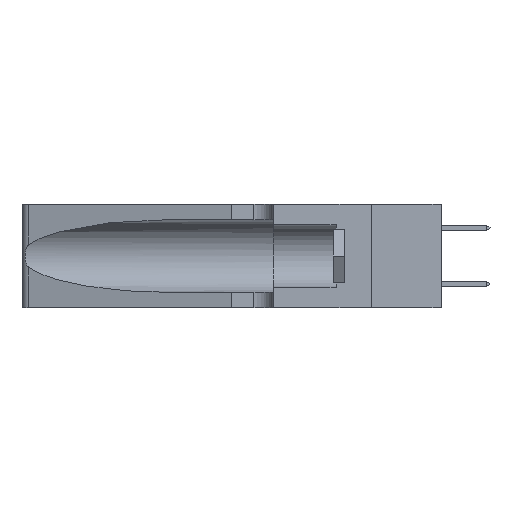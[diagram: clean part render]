
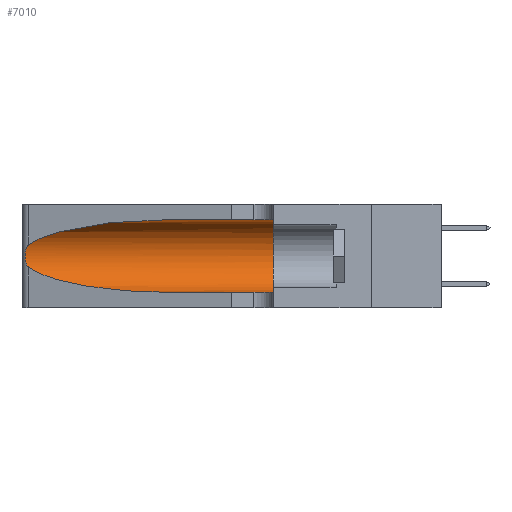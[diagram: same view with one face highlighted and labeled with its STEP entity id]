
A CAD part, left-side view. The second image highlights one B-rep face of the part: STEP entity #7010.
In plain terms, the highlighted cylindrical face has radius 3.308 mm (diameter 6.617 mm), a partial arc.
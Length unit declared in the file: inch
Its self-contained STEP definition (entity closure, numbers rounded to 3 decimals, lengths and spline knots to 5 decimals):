
#22 = CARTESIAN_POINT ( 'NONE',  ( 0.26017, 1.23833, 0.17102 ) ) ;
#208 = ORIENTED_EDGE ( 'NONE', *, *, #18053, .T. ) ;
#286 = VERTEX_POINT ( 'NONE', #5346 ) ;
#726 = EDGE_CURVE ( 'NONE', #14217, #21030, #21893, .T. ) ;
#1141 =( BOUNDED_CURVE ( )  B_SPLINE_CURVE ( 3, ( #11148, #11745, #5069, #12474 ),
 .UNSPECIFIED., .F., .F. ) 
 B_SPLINE_CURVE_WITH_KNOTS ( ( 4, 4 ),
 ( 3.44316, 4.71239 ),
 .UNSPECIFIED. ) 
 CURVE ( )  GEOMETRIC_REPRESENTATION_ITEM ( )  RATIONAL_B_SPLINE_CURVE ( ( 1., 0.87, 0.87, 1. ) ) 
 REPRESENTATION_ITEM ( '' )  );
#1900 = CARTESIAN_POINT ( 'NONE',  ( 0.25787, 1.23484, 0.2124 ) ) ;
#2143 = CARTESIAN_POINT ( 'NONE',  ( 0.26075, 1.23896, 0.19203 ) ) ;
#2318 = VERTEX_POINT ( 'NONE', #16138 ) ;
#2430 = EDGE_CURVE ( 'NONE', #21030, #9475, #13844, .T. ) ;
#3172 = CARTESIAN_POINT ( 'NONE',  ( 0.25487, 1.22718, 0.22369 ) ) ;
#3685 = CARTESIAN_POINT ( 'NONE',  ( 0.25856, 1.23593, 0.16098 ) ) ;
#3752 = CARTESIAN_POINT ( 'NONE',  ( 0.25854, 1.2359, 0.20912 ) ) ;
#3926 = CARTESIAN_POINT ( 'NONE',  ( 0.1305, 0.72297, 0.31525 ) ) ;
#4251 = CARTESIAN_POINT ( 'NONE',  ( 0.25555, 1.22993, 0.14849 ) ) ;
#4576 = CARTESIAN_POINT ( 'NONE',  ( 0.1305, 1.61858, 0.185 ) ) ;
#4674 = ORIENTED_EDGE ( 'NONE', *, *, #5814, .T. ) ;
#4937 = CARTESIAN_POINT ( 'NONE',  ( 0.1305, 1.61858, 0.05475 ) ) ;
#5069 = CARTESIAN_POINT ( 'NONE',  ( 0.18966, 0.96281, 0.05475 ) ) ;
#5147 = EDGE_CURVE ( 'NONE', #286, #2318, #13056, .T. ) ;
#5334 = ORIENTED_EDGE ( 'NONE', *, *, #726, .T. ) ;
#5346 = CARTESIAN_POINT ( 'NONE',  ( 0.1305, 0.35, 0.31525 ) ) ;
#5475 = CARTESIAN_POINT ( 'NONE',  ( 0.2373, 1.15595, 0.28018 ) ) ;
#5515 = CARTESIAN_POINT ( 'NONE',  ( 0.25639, 1.23186, 0.15144 ) ) ;
#5814 = EDGE_CURVE ( 'NONE', #9475, #20450, #1141, .T. ) ;
#7010 = ADVANCED_FACE ( 'NONE', ( #17725 ), #16024, .F. ) ;
#7580 = CARTESIAN_POINT ( 'NONE',  ( 0.25487, 1.22718, 0.22369 ) ) ;
#7705 = CARTESIAN_POINT ( 'NONE',  ( 0.25487, 1.22718, 0.14631 ) ) ;
#8514 = DIRECTION ( 'NONE',  ( 0., -1., 0. ) ) ;
#8834 = LINE ( 'NONE', #20556, #15695 ) ;
#8961 = CARTESIAN_POINT ( 'NONE',  ( 0.1305, 0.72297, 0.31525 ) ) ;
#9475 = VERTEX_POINT ( 'NONE', #7705 ) ;
#10268 = DIRECTION ( 'NONE',  ( 0., 0., 1. ) ) ;
#10344 = DIRECTION ( 'NONE',  ( 0., 1., 0. ) ) ;
#10868 = CARTESIAN_POINT ( 'NONE',  ( 0.25555, 1.22994, 0.2215 ) ) ;
#11148 = CARTESIAN_POINT ( 'NONE',  ( 0.25487, 1.22718, 0.14631 ) ) ;
#11170 = CARTESIAN_POINT ( 'NONE',  ( 0.26018, 1.23835, 0.19895 ) ) ;
#11745 = CARTESIAN_POINT ( 'NONE',  ( 0.2373, 1.15595, 0.08982 ) ) ;
#11842 = CARTESIAN_POINT ( 'NONE',  ( 0.25487, 1.22718, 0.14631 ) ) ;
#12474 = CARTESIAN_POINT ( 'NONE',  ( 0.1305, 0.72297, 0.05475 ) ) ;
#13056 = CIRCLE ( 'NONE', #15812, 0.13025 ) ;
#13256 = CARTESIAN_POINT ( 'NONE',  ( 0.1305, 0.72297, 0.05475 ) ) ;
#13257 = DIRECTION ( 'NONE',  ( 0., -1., 0. ) ) ;
#13844 = B_SPLINE_CURVE_WITH_KNOTS ( 'NONE', 3,
 ( #7580, #10868, #22161, #1900, #3752, #11170, #2143, #21847, #22, #3685, #16455, #5515, #4251, #11842 ),
 .UNSPECIFIED., .F., .F.,
 ( 4, 2, 2, 2, 2, 2, 4 ),
 ( 0., 0.00027, 0.00053, 0.00107, 0.0016, 0.00187, 0.00214 ),
 .UNSPECIFIED. ) ;
#14217 = VERTEX_POINT ( 'NONE', #3926 ) ;
#15176 = ORIENTED_EDGE ( 'NONE', *, *, #2430, .T. ) ;
#15252 = EDGE_LOOP ( 'NONE', ( #5334, #15176, #4674, #208, #22486, #15379 ) ) ;
#15379 = ORIENTED_EDGE ( 'NONE', *, *, #17724, .F. ) ;
#15695 = VECTOR ( 'NONE', #13257, 39.37008 ) ;
#15812 = AXIS2_PLACEMENT_3D ( 'NONE', #19545, #10344, #10268 ) ;
#16024 = CYLINDRICAL_SURFACE ( 'NONE', #16303, 0.13025 ) ;
#16138 = CARTESIAN_POINT ( 'NONE',  ( 0.1305, 0.35, 0.05475 ) ) ;
#16303 = AXIS2_PLACEMENT_3D ( 'NONE', #4576, #20918, #22941 ) ;
#16455 = CARTESIAN_POINT ( 'NONE',  ( 0.25789, 1.23486, 0.15765 ) ) ;
#16554 = CARTESIAN_POINT ( 'NONE',  ( 0.25487, 1.22718, 0.22369 ) ) ;
#17724 = EDGE_CURVE ( 'NONE', #14217, #286, #8834, .T. ) ;
#17725 = FACE_OUTER_BOUND ( 'NONE', #15252, .T. ) ;
#17948 = LINE ( 'NONE', #4937, #19380 ) ;
#18053 = EDGE_CURVE ( 'NONE', #20450, #2318, #17948, .T. ) ;
#19380 = VECTOR ( 'NONE', #8514, 39.37008 ) ;
#19545 = CARTESIAN_POINT ( 'NONE',  ( 0.1305, 0.35, 0.185 ) ) ;
#20450 = VERTEX_POINT ( 'NONE', #13256 ) ;
#20556 = CARTESIAN_POINT ( 'NONE',  ( 0.1305, 1.61858, 0.31525 ) ) ;
#20918 = DIRECTION ( 'NONE',  ( 0., -1., 0. ) ) ;
#21030 = VERTEX_POINT ( 'NONE', #16554 ) ;
#21723 = CARTESIAN_POINT ( 'NONE',  ( 0.18966, 0.96281, 0.31525 ) ) ;
#21847 = CARTESIAN_POINT ( 'NONE',  ( 0.26075, 1.23896, 0.178 ) ) ;
#21893 =( BOUNDED_CURVE ( )  B_SPLINE_CURVE ( 3, ( #8961, #21723, #5475, #3172 ),
 .UNSPECIFIED., .F., .F. ) 
 B_SPLINE_CURVE_WITH_KNOTS ( ( 4, 4 ),
 ( 1.5708, 2.84003 ),
 .UNSPECIFIED. ) 
 CURVE ( )  GEOMETRIC_REPRESENTATION_ITEM ( )  RATIONAL_B_SPLINE_CURVE ( ( 1., 0.87, 0.87, 1. ) ) 
 REPRESENTATION_ITEM ( '' )  );
#22161 = CARTESIAN_POINT ( 'NONE',  ( 0.25639, 1.23184, 0.21858 ) ) ;
#22486 = ORIENTED_EDGE ( 'NONE', *, *, #5147, .F. ) ;
#22941 = DIRECTION ( 'NONE',  ( 0., 0., -1. ) ) ;
